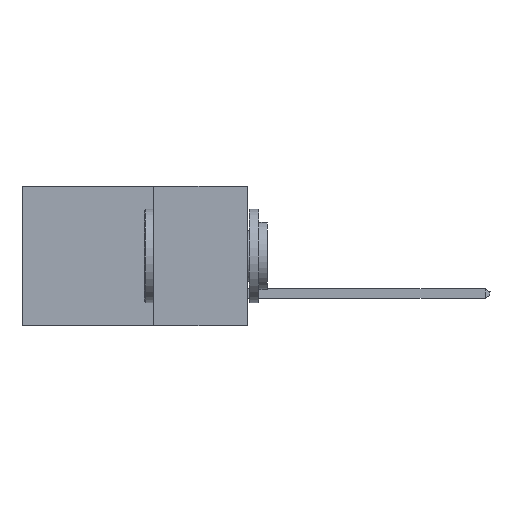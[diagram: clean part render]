
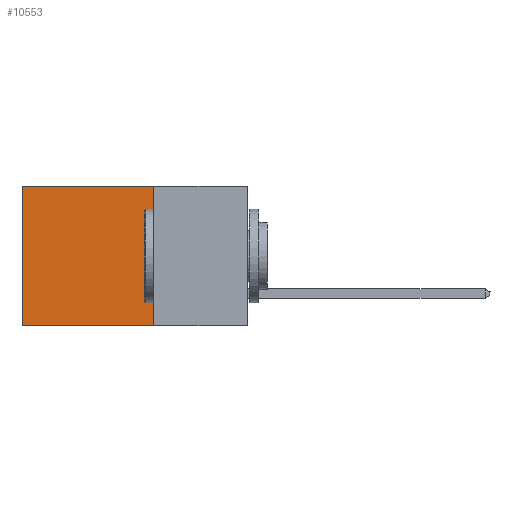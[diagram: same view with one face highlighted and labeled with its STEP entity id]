
A CAD part, left-side view. The second image highlights one B-rep face of the part: STEP entity #10553.
In plain terms, the highlighted planar face has unit normal (-1, 0, 0).
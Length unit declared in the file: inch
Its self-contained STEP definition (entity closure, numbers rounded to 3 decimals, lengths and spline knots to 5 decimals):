
#47 = CARTESIAN_POINT ( 'NONE',  ( 0.2615, 0.25, -0.37 ) ) ;
#77 = CARTESIAN_POINT ( 'NONE',  ( 0.2615, 0.25, -0.37 ) ) ;
#125 = VECTOR ( 'NONE', #10639, 39.37008 ) ;
#370 = DIRECTION ( 'NONE',  ( 0., 1., 0. ) ) ;
#568 = AXIS2_PLACEMENT_3D ( 'NONE', #47, #1038, #2800 ) ;
#957 = CARTESIAN_POINT ( 'NONE',  ( 0.2615, 0.6, 0. ) ) ;
#1038 = DIRECTION ( 'NONE',  ( 1., 0., 0. ) ) ;
#1499 = EDGE_CURVE ( 'NONE', #6213, #9132, #2123, .T. ) ;
#1772 = EDGE_LOOP ( 'NONE', ( #10022, #6123, #3975, #4957 ) ) ;
#2123 = LINE ( 'NONE', #6230, #10397 ) ;
#2498 = DIRECTION ( 'NONE',  ( 0., 0., -1. ) ) ;
#2759 = CARTESIAN_POINT ( 'NONE',  ( 0.2615, 0.6, -0.37 ) ) ;
#2800 = DIRECTION ( 'NONE',  ( 0., 0., -1. ) ) ;
#3083 = DIRECTION ( 'NONE',  ( 0., 0., -1. ) ) ;
#3117 = EDGE_CURVE ( 'NONE', #9132, #7291, #3595, .T. ) ;
#3277 = EDGE_CURVE ( 'NONE', #6213, #9680, #6866, .T. ) ;
#3448 = CARTESIAN_POINT ( 'NONE',  ( 0.2615, 0.6, -0.37 ) ) ;
#3595 = LINE ( 'NONE', #2759, #11492 ) ;
#3975 = ORIENTED_EDGE ( 'NONE', *, *, #3277, .F. ) ;
#4957 = ORIENTED_EDGE ( 'NONE', *, *, #1499, .T. ) ;
#4999 = PLANE ( 'NONE',  #568 ) ;
#6069 = EDGE_CURVE ( 'NONE', #9680, #7291, #6598, .T. ) ;
#6123 = ORIENTED_EDGE ( 'NONE', *, *, #6069, .F. ) ;
#6213 = VERTEX_POINT ( 'NONE', #6295 ) ;
#6230 = CARTESIAN_POINT ( 'NONE',  ( 0.2615, 0.25, 0. ) ) ;
#6295 = CARTESIAN_POINT ( 'NONE',  ( 0.2615, 0.25, 0. ) ) ;
#6598 = LINE ( 'NONE', #10542, #125 ) ;
#6866 = LINE ( 'NONE', #77, #12330 ) ;
#7193 = CARTESIAN_POINT ( 'NONE',  ( 0.2615, 0.25, -0.37 ) ) ;
#7291 = VERTEX_POINT ( 'NONE', #3448 ) ;
#9132 = VERTEX_POINT ( 'NONE', #957 ) ;
#9680 = VERTEX_POINT ( 'NONE', #7193 ) ;
#10022 = ORIENTED_EDGE ( 'NONE', *, *, #3117, .T. ) ;
#10397 = VECTOR ( 'NONE', #370, 39.37008 ) ;
#10542 = CARTESIAN_POINT ( 'NONE',  ( 0.2615, 0.25, -0.37 ) ) ;
#10553 = ADVANCED_FACE ( 'NONE', ( #11823 ), #4999, .F. ) ;
#10639 = DIRECTION ( 'NONE',  ( 0., 1., 0. ) ) ;
#11492 = VECTOR ( 'NONE', #2498, 39.37008 ) ;
#11823 = FACE_OUTER_BOUND ( 'NONE', #1772, .T. ) ;
#12330 = VECTOR ( 'NONE', #3083, 39.37008 ) ;
